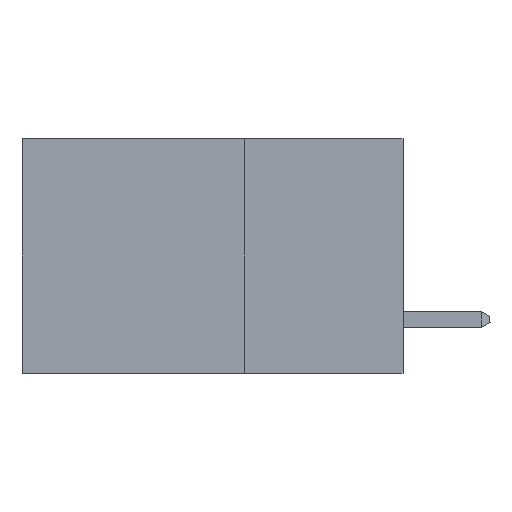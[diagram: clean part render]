
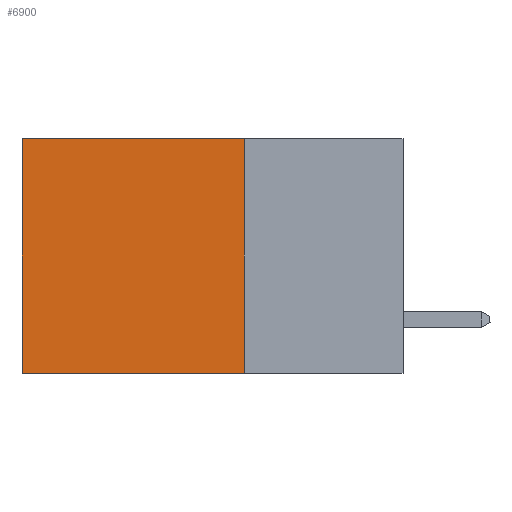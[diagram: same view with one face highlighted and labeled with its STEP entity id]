
A CAD part, left-side view. The second image highlights one B-rep face of the part: STEP entity #6900.
In plain terms, the highlighted planar face has unit normal (-1, 0, 0).
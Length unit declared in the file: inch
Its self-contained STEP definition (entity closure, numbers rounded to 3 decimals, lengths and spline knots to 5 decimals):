
#800 = CARTESIAN_POINT ( 'NONE',  ( 0.2875, 0.6, 0. ) ) ;
#810 = FACE_OUTER_BOUND ( 'NONE', #1147, .T. ) ;
#1147 = EDGE_LOOP ( 'NONE', ( #15147, #6314, #16415, #14559 ) ) ;
#1388 = VECTOR ( 'NONE', #14596, 39.37008 ) ;
#3845 = VECTOR ( 'NONE', #12594, 39.37008 ) ;
#3899 = VECTOR ( 'NONE', #15195, 39.37008 ) ;
#3909 = VERTEX_POINT ( 'NONE', #15720 ) ;
#5841 = PLANE ( 'NONE',  #12073 ) ;
#5866 = DIRECTION ( 'NONE',  ( 0., 1., 0. ) ) ;
#6314 = ORIENTED_EDGE ( 'NONE', *, *, #16117, .F. ) ;
#6751 = CARTESIAN_POINT ( 'NONE',  ( 0.2875, 0.6, 0. ) ) ;
#6900 = ADVANCED_FACE ( 'NONE', ( #810 ), #5841, .F. ) ;
#7566 = EDGE_CURVE ( 'NONE', #8512, #3909, #12712, .T. ) ;
#7635 = CARTESIAN_POINT ( 'NONE',  ( 0.2875, 0.25, -0.37 ) ) ;
#8218 = CARTESIAN_POINT ( 'NONE',  ( 0.2875, 0.25, 0. ) ) ;
#8512 = VERTEX_POINT ( 'NONE', #6751 ) ;
#8799 = DIRECTION ( 'NONE',  ( 0., 0., -1. ) ) ;
#9185 = CARTESIAN_POINT ( 'NONE',  ( 0.2875, 0.25, 0. ) ) ;
#9410 = CARTESIAN_POINT ( 'NONE',  ( 0.2875, 0.25, -0.37 ) ) ;
#9784 = EDGE_CURVE ( 'NONE', #18269, #8512, #11346, .T. ) ;
#10193 = CARTESIAN_POINT ( 'NONE',  ( 0.2875, 0.25, 0. ) ) ;
#10893 = VECTOR ( 'NONE', #5866, 39.37008 ) ;
#11346 = LINE ( 'NONE', #17290, #10893 ) ;
#11875 = EDGE_CURVE ( 'NONE', #18269, #17598, #14235, .T. ) ;
#12073 = AXIS2_PLACEMENT_3D ( 'NONE', #10193, #15929, #8799 ) ;
#12594 = DIRECTION ( 'NONE',  ( 0., 0., -1. ) ) ;
#12712 = LINE ( 'NONE', #800, #3899 ) ;
#14235 = LINE ( 'NONE', #8218, #3845 ) ;
#14559 = ORIENTED_EDGE ( 'NONE', *, *, #9784, .T. ) ;
#14596 = DIRECTION ( 'NONE',  ( 0., 1., 0. ) ) ;
#15147 = ORIENTED_EDGE ( 'NONE', *, *, #7566, .T. ) ;
#15195 = DIRECTION ( 'NONE',  ( 0., 0., -1. ) ) ;
#15720 = CARTESIAN_POINT ( 'NONE',  ( 0.2875, 0.6, -0.37 ) ) ;
#15929 = DIRECTION ( 'NONE',  ( 1., 0., 0. ) ) ;
#16117 = EDGE_CURVE ( 'NONE', #17598, #3909, #16689, .T. ) ;
#16415 = ORIENTED_EDGE ( 'NONE', *, *, #11875, .F. ) ;
#16689 = LINE ( 'NONE', #7635, #1388 ) ;
#17290 = CARTESIAN_POINT ( 'NONE',  ( 0.2875, 0.25, 0. ) ) ;
#17598 = VERTEX_POINT ( 'NONE', #9410 ) ;
#18269 = VERTEX_POINT ( 'NONE', #9185 ) ;
